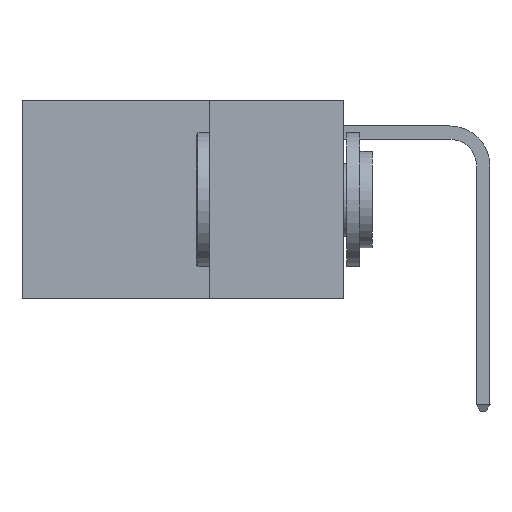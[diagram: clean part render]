
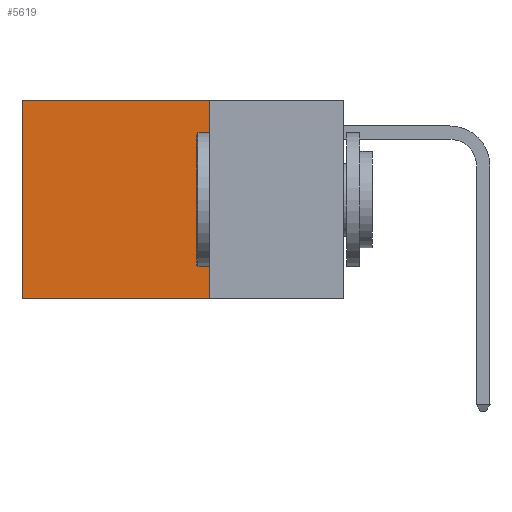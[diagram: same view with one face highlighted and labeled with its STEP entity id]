
A CAD part, left-side view. The second image highlights one B-rep face of the part: STEP entity #5619.
In plain terms, the highlighted planar face has unit normal (-1, 0, 0).
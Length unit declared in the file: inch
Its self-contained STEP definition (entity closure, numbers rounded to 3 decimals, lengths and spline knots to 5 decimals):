
#47 = EDGE_LOOP ( 'NONE', ( #6704, #5669, #3752, #5382 ) ) ;
#74 = VERTEX_POINT ( 'NONE', #1392 ) ;
#454 = CARTESIAN_POINT ( 'NONE',  ( 0.2625, 0.25, 0. ) ) ;
#1157 = DIRECTION ( 'NONE',  ( 0., 0., -1. ) ) ;
#1328 = EDGE_CURVE ( 'NONE', #7165, #74, #9728, .T. ) ;
#1392 = CARTESIAN_POINT ( 'NONE',  ( 0.2625, 0.6, -0.37 ) ) ;
#2288 = EDGE_CURVE ( 'NONE', #8907, #74, #6656, .T. ) ;
#2527 = CARTESIAN_POINT ( 'NONE',  ( 0.2625, 0.25, 0. ) ) ;
#2533 = AXIS2_PLACEMENT_3D ( 'NONE', #454, #6396, #1157 ) ;
#2916 = EDGE_CURVE ( 'NONE', #4982, #7165, #4924, .T. ) ;
#3752 = ORIENTED_EDGE ( 'NONE', *, *, #2916, .F. ) ;
#4924 = LINE ( 'NONE', #2527, #4941 ) ;
#4941 = VECTOR ( 'NONE', #7855, 39.37008 ) ;
#4981 = CARTESIAN_POINT ( 'NONE',  ( 0.2625, 0.25, 0. ) ) ;
#4982 = VERTEX_POINT ( 'NONE', #4981 ) ;
#5020 = CARTESIAN_POINT ( 'NONE',  ( 0.2625, 0.25, 0. ) ) ;
#5042 = VECTOR ( 'NONE', #5901, 39.37008 ) ;
#5095 = LINE ( 'NONE', #5020, #5042 ) ;
#5237 = FACE_OUTER_BOUND ( 'NONE', #47, .T. ) ;
#5382 = ORIENTED_EDGE ( 'NONE', *, *, #5696, .T. ) ;
#5501 = DIRECTION ( 'NONE',  ( 0., 1., 0. ) ) ;
#5619 = ADVANCED_FACE ( 'NONE', ( #5237 ), #8533, .F. ) ;
#5669 = ORIENTED_EDGE ( 'NONE', *, *, #1328, .F. ) ;
#5696 = EDGE_CURVE ( 'NONE', #4982, #8907, #5095, .T. ) ;
#5706 = CARTESIAN_POINT ( 'NONE',  ( 0.2625, 0.25, -0.37 ) ) ;
#5901 = DIRECTION ( 'NONE',  ( 0., 1., 0. ) ) ;
#6396 = DIRECTION ( 'NONE',  ( 1., 0., 0. ) ) ;
#6414 = CARTESIAN_POINT ( 'NONE',  ( 0.2625, 0.25, -0.37 ) ) ;
#6656 = LINE ( 'NONE', #8914, #6764 ) ;
#6704 = ORIENTED_EDGE ( 'NONE', *, *, #2288, .T. ) ;
#6764 = VECTOR ( 'NONE', #7401, 39.37008 ) ;
#7165 = VERTEX_POINT ( 'NONE', #6414 ) ;
#7401 = DIRECTION ( 'NONE',  ( 0., 0., -1. ) ) ;
#7855 = DIRECTION ( 'NONE',  ( 0., 0., -1. ) ) ;
#8533 = PLANE ( 'NONE',  #2533 ) ;
#8907 = VERTEX_POINT ( 'NONE', #9296 ) ;
#8914 = CARTESIAN_POINT ( 'NONE',  ( 0.2625, 0.6, 0. ) ) ;
#9296 = CARTESIAN_POINT ( 'NONE',  ( 0.2625, 0.6, 0. ) ) ;
#9707 = VECTOR ( 'NONE', #5501, 39.37008 ) ;
#9728 = LINE ( 'NONE', #5706, #9707 ) ;
